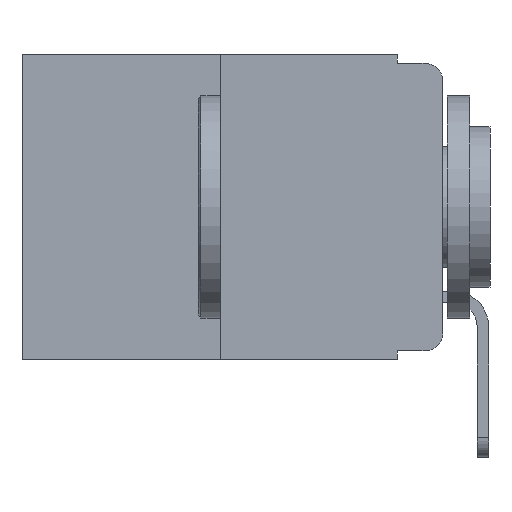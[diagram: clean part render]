
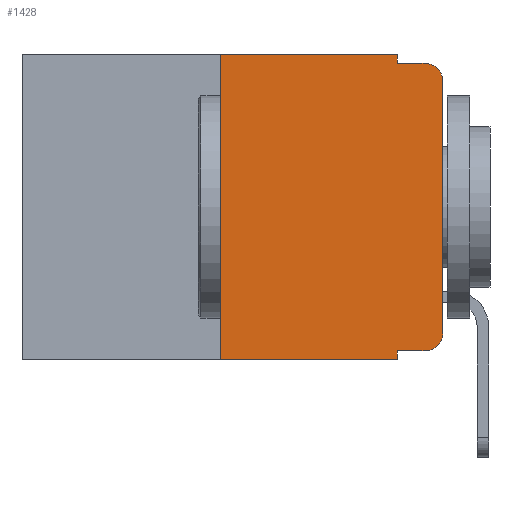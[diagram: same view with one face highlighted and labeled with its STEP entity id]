
A CAD part, left-side view. The second image highlights one B-rep face of the part: STEP entity #1428.
In plain terms, the highlighted planar face has unit normal (-1, 0, 0).
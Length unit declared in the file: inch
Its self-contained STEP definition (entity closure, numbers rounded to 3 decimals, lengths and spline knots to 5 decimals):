
#150 = CARTESIAN_POINT ( 'NONE',  ( 0., 0.25, -0.343 ) ) ;
#417 = DIRECTION ( 'NONE',  ( 0., 0., 1. ) ) ;
#443 = ORIENTED_EDGE ( 'NONE', *, *, #6995, .T. ) ;
#602 = VERTEX_POINT ( 'NONE', #150 ) ;
#789 = ORIENTED_EDGE ( 'NONE', *, *, #7573, .T. ) ;
#1143 = ORIENTED_EDGE ( 'NONE', *, *, #5950, .F. ) ;
#1428 = ADVANCED_FACE ( 'NONE', ( #3671 ), #6835, .F. ) ;
#1456 = LINE ( 'NONE', #7557, #6758 ) ;
#1497 = LINE ( 'NONE', #12948, #7102 ) ;
#1644 = CARTESIAN_POINT ( 'NONE',  ( 0., 0.02, -0.313 ) ) ;
#1692 = ORIENTED_EDGE ( 'NONE', *, *, #9939, .F. ) ;
#1724 = DIRECTION ( 'NONE',  ( 0., 0., -1. ) ) ;
#1779 = ORIENTED_EDGE ( 'NONE', *, *, #13401, .F. ) ;
#1876 = VERTEX_POINT ( 'NONE', #12224 ) ;
#2150 = AXIS2_PLACEMENT_3D ( 'NONE', #5609, #12496, #6684 ) ;
#2514 = AXIS2_PLACEMENT_3D ( 'NONE', #1644, #9220, #2828 ) ;
#2593 = CARTESIAN_POINT ( 'NONE',  ( 0., 0.051, -0.333 ) ) ;
#2651 = LINE ( 'NONE', #8789, #5309 ) ;
#2815 = DIRECTION ( 'NONE',  ( 0., 0., -1. ) ) ;
#2828 = DIRECTION ( 'NONE',  ( 0., 0., -1. ) ) ;
#2993 = VERTEX_POINT ( 'NONE', #6053 ) ;
#3150 = ORIENTED_EDGE ( 'NONE', *, *, #10276, .F. ) ;
#3250 = ORIENTED_EDGE ( 'NONE', *, *, #9549, .F. ) ;
#3387 = VERTEX_POINT ( 'NONE', #10804 ) ;
#3497 = DIRECTION ( 'NONE',  ( 0., -1., 0. ) ) ;
#3671 = FACE_OUTER_BOUND ( 'NONE', #5249, .T. ) ;
#3785 = LINE ( 'NONE', #8310, #11543 ) ;
#3794 = CIRCLE ( 'NONE', #2150, 0.02 ) ;
#4268 = CARTESIAN_POINT ( 'NONE',  ( 0., 0.051, -0.333 ) ) ;
#4424 = VERTEX_POINT ( 'NONE', #4705 ) ;
#4475 = LINE ( 'NONE', #13329, #6965 ) ;
#4544 = EDGE_CURVE ( 'NONE', #4668, #8535, #8412, .T. ) ;
#4668 = VERTEX_POINT ( 'NONE', #4268 ) ;
#4705 = CARTESIAN_POINT ( 'NONE',  ( 0., 0.051, -0.01 ) ) ;
#5249 = EDGE_LOOP ( 'NONE', ( #11414, #8467, #3150, #1779, #3250, #1143, #443, #1692, #12059, #789 ) ) ;
#5309 = VECTOR ( 'NONE', #3497, 39.37008 ) ;
#5480 = DIRECTION ( 'NONE',  ( 1., 0., 0. ) ) ;
#5552 = CARTESIAN_POINT ( 'NONE',  ( 0., 0.02, -0.333 ) ) ;
#5609 = CARTESIAN_POINT ( 'NONE',  ( 0., 0.02, -0.03 ) ) ;
#5950 = EDGE_CURVE ( 'NONE', #602, #1876, #1497, .T. ) ;
#6053 = CARTESIAN_POINT ( 'NONE',  ( 0., 0.051, -0.343 ) ) ;
#6189 = DIRECTION ( 'NONE',  ( 0., -1., 0. ) ) ;
#6684 = DIRECTION ( 'NONE',  ( 0., 0., -1. ) ) ;
#6758 = VECTOR ( 'NONE', #13255, 39.37008 ) ;
#6835 = PLANE ( 'NONE',  #10121 ) ;
#6965 = VECTOR ( 'NONE', #8662, 39.37008 ) ;
#6995 = EDGE_CURVE ( 'NONE', #602, #2993, #1456, .T. ) ;
#7102 = VECTOR ( 'NONE', #417, 39.37008 ) ;
#7557 = CARTESIAN_POINT ( 'NONE',  ( 0., 0.473, -0.343 ) ) ;
#7573 = EDGE_CURVE ( 'NONE', #8535, #7734, #8188, .T. ) ;
#7734 = VERTEX_POINT ( 'NONE', #10361 ) ;
#7895 = DIRECTION ( 'NONE',  ( 0., 0., -1. ) ) ;
#8188 = CIRCLE ( 'NONE', #2514, 0.02 ) ;
#8310 = CARTESIAN_POINT ( 'NONE',  ( 0., 0.051, 0. ) ) ;
#8412 = LINE ( 'NONE', #2593, #10947 ) ;
#8417 = CARTESIAN_POINT ( 'NONE',  ( 0., 0.473, 0. ) ) ;
#8467 = ORIENTED_EDGE ( 'NONE', *, *, #9491, .T. ) ;
#8535 = VERTEX_POINT ( 'NONE', #5552 ) ;
#8603 = LINE ( 'NONE', #9673, #13292 ) ;
#8662 = DIRECTION ( 'NONE',  ( 0., -1., 0. ) ) ;
#8681 = EDGE_CURVE ( 'NONE', #7734, #13018, #8603, .T. ) ;
#8789 = CARTESIAN_POINT ( 'NONE',  ( 0., 0.473, 0. ) ) ;
#9220 = DIRECTION ( 'NONE',  ( -1., 0., 0. ) ) ;
#9312 = CARTESIAN_POINT ( 'NONE',  ( 0., 0.02, -0.01 ) ) ;
#9491 = EDGE_CURVE ( 'NONE', #13018, #11249, #3794, .T. ) ;
#9549 = EDGE_CURVE ( 'NONE', #1876, #3387, #2651, .T. ) ;
#9673 = CARTESIAN_POINT ( 'NONE',  ( 0., 0., 0. ) ) ;
#9939 = EDGE_CURVE ( 'NONE', #4668, #2993, #3785, .T. ) ;
#10121 = AXIS2_PLACEMENT_3D ( 'NONE', #8417, #5480, #2815 ) ;
#10276 = EDGE_CURVE ( 'NONE', #4424, #11249, #4475, .T. ) ;
#10361 = CARTESIAN_POINT ( 'NONE',  ( 0., 0., -0.313 ) ) ;
#10449 = LINE ( 'NONE', #12635, #13219 ) ;
#10631 = DIRECTION ( 'NONE',  ( 0., 0., 1. ) ) ;
#10804 = CARTESIAN_POINT ( 'NONE',  ( 0., 0.051, 0. ) ) ;
#10947 = VECTOR ( 'NONE', #6189, 39.37008 ) ;
#11249 = VERTEX_POINT ( 'NONE', #9312 ) ;
#11414 = ORIENTED_EDGE ( 'NONE', *, *, #8681, .T. ) ;
#11543 = VECTOR ( 'NONE', #1724, 39.37008 ) ;
#12059 = ORIENTED_EDGE ( 'NONE', *, *, #4544, .T. ) ;
#12224 = CARTESIAN_POINT ( 'NONE',  ( 0., 0.25, 0. ) ) ;
#12496 = DIRECTION ( 'NONE',  ( -1., 0., 0. ) ) ;
#12635 = CARTESIAN_POINT ( 'NONE',  ( 0., 0.051, 0. ) ) ;
#12948 = CARTESIAN_POINT ( 'NONE',  ( 0., 0.25, 0. ) ) ;
#13018 = VERTEX_POINT ( 'NONE', #13030 ) ;
#13030 = CARTESIAN_POINT ( 'NONE',  ( 0., 0., -0.03 ) ) ;
#13219 = VECTOR ( 'NONE', #7895, 39.37008 ) ;
#13255 = DIRECTION ( 'NONE',  ( 0., -1., 0. ) ) ;
#13292 = VECTOR ( 'NONE', #10631, 39.37008 ) ;
#13329 = CARTESIAN_POINT ( 'NONE',  ( 0., 0.051, -0.01 ) ) ;
#13401 = EDGE_CURVE ( 'NONE', #3387, #4424, #10449, .T. ) ;
